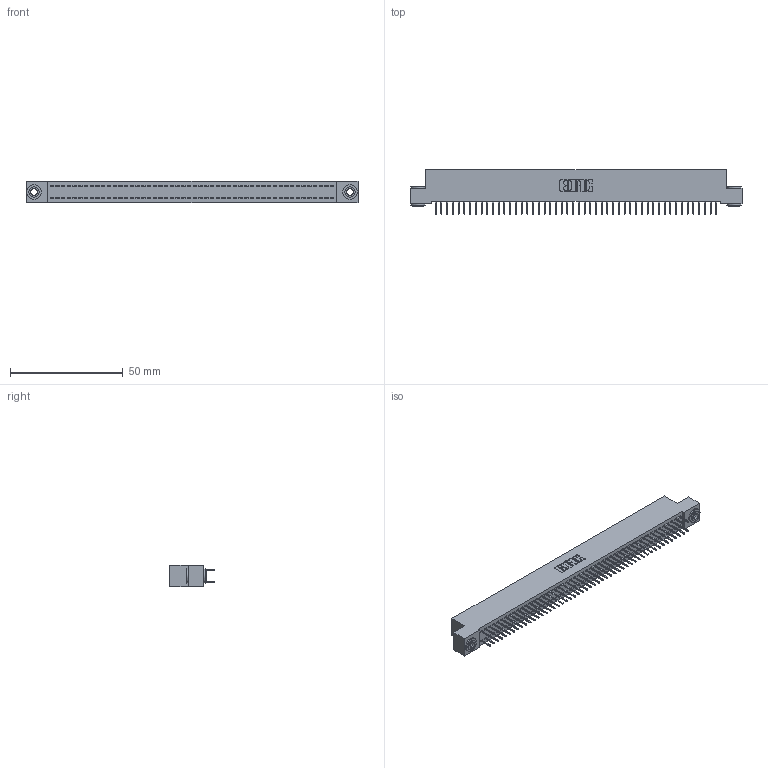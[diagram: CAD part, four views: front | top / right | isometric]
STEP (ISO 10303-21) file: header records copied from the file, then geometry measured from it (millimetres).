
FILE_DESCRIPTION (( 'STEP AP203' ), '1' );
FILE_NAME ('392-100-524-203.STEP', '2018-08-18T18:12:16', ( '' ), ( '' ), 'SwSTEP 2.0', 'SolidWorks 2016', '' );
FILE_SCHEMA (( 'CONFIG_CONTROL_DESIGN' ));
Length unit declared in the file: inch
Products named in the file (4): 342 Part_.156 TH; 345-292-001_345-293-124; 342-250-002_345-250-002-102; 392-100-524-203
Assembly tree (103 placements, depth 2):
  392-100-524-203
    342 Part_.156 TH
    345-292-001_345-293-124  x100
    342-250-002_345-250-002-102  x2
Bounding box: 147.32 x 19.69 x 9.4 mm (x, y, z)
Volume: 13146 mm3; surface area: 21416 mm2
Topology: 103 solids, 103 shells, 5748 faces, 16275 edges, 10446 vertices
Faces by surface type: plane 4276, cylinder 1464, cone 8
Entity records: 31724 total; most frequent: CARTESIAN_POINT 5221, ORIENTED_EDGE 5150, DIRECTION 4481, EDGE_CURVE 2575, VECTOR 2427, LINE 2427, VERTEX_POINT 1710, AXIS2_PLACEMENT_3D 1027
